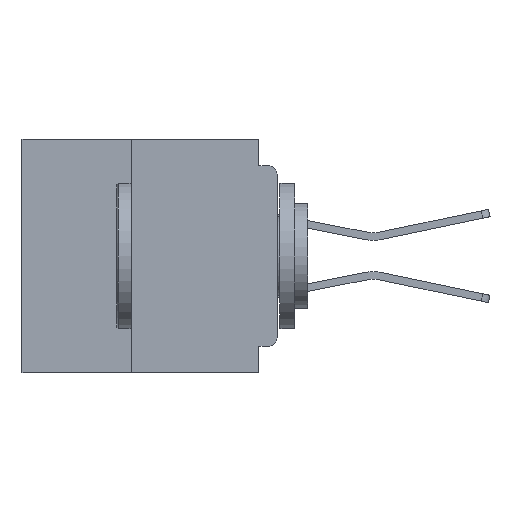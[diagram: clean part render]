
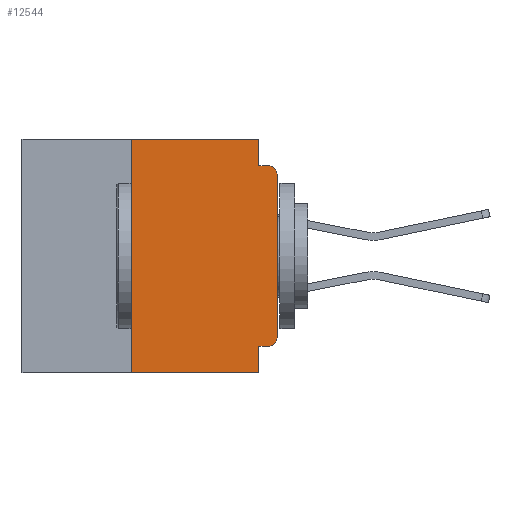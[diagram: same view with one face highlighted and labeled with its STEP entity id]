
A CAD part, left-side view. The second image highlights one B-rep face of the part: STEP entity #12544.
In plain terms, the highlighted planar face has unit normal (-1, 0, 0).
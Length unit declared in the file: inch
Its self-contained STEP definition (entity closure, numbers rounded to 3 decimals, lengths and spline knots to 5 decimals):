
#443 = CARTESIAN_POINT ( 'NONE',  ( 0., 0.015, -0.045 ) ) ;
#712 = LINE ( 'NONE', #4609, #33017 ) ;
#1486 = VECTOR ( 'NONE', #48933, 39.37008 ) ;
#1569 = VERTEX_POINT ( 'NONE', #37169 ) ;
#1986 = LINE ( 'NONE', #53077, #34319 ) ;
#2642 = ORIENTED_EDGE ( 'NONE', *, *, #38864, .F. ) ;
#3159 = CARTESIAN_POINT ( 'NONE',  ( 0., 0.25, -0.4 ) ) ;
#4357 = EDGE_CURVE ( 'NONE', #14208, #6623, #23894, .T. ) ;
#4609 = CARTESIAN_POINT ( 'NONE',  ( 0., 0., -0.045 ) ) ;
#4892 = VECTOR ( 'NONE', #44281, 39.37008 ) ;
#4979 = PLANE ( 'NONE',  #53976 ) ;
#5195 = CARTESIAN_POINT ( 'NONE',  ( 0., 0.031, -0.4 ) ) ;
#5841 = LINE ( 'NONE', #3159, #26900 ) ;
#6285 = LINE ( 'NONE', #45134, #27344 ) ;
#6504 = DIRECTION ( 'NONE',  ( 0., -1., 0. ) ) ;
#6623 = VERTEX_POINT ( 'NONE', #23574 ) ;
#7063 = CARTESIAN_POINT ( 'NONE',  ( 0., 0.031, -0.045 ) ) ;
#9171 = DIRECTION ( 'NONE',  ( -1., 0., 0. ) ) ;
#9175 = DIRECTION ( 'NONE',  ( 1., 0., 0. ) ) ;
#9503 = AXIS2_PLACEMENT_3D ( 'NONE', #43676, #18572, #47808 ) ;
#9841 = VERTEX_POINT ( 'NONE', #47493 ) ;
#10093 = CIRCLE ( 'NONE', #31548, 0.015 ) ;
#10933 = LINE ( 'NONE', #52567, #20792 ) ;
#11069 = ORIENTED_EDGE ( 'NONE', *, *, #26938, .F. ) ;
#12544 = ADVANCED_FACE ( 'NONE', ( #17774 ), #4979, .F. ) ;
#14208 = VERTEX_POINT ( 'NONE', #30816 ) ;
#14665 = ORIENTED_EDGE ( 'NONE', *, *, #43760, .T. ) ;
#15683 = DIRECTION ( 'NONE',  ( 0., 0., -1. ) ) ;
#16078 = LINE ( 'NONE', #40125, #4892 ) ;
#16289 = EDGE_CURVE ( 'NONE', #6623, #36431, #1986, .T. ) ;
#17478 = CARTESIAN_POINT ( 'NONE',  ( 0., 0.437, 0. ) ) ;
#17774 = FACE_OUTER_BOUND ( 'NONE', #49546, .T. ) ;
#18572 = DIRECTION ( 'NONE',  ( -1., 0., 0. ) ) ;
#19112 = EDGE_CURVE ( 'NONE', #25032, #36431, #6285, .T. ) ;
#19873 = VERTEX_POINT ( 'NONE', #40147 ) ;
#20771 = VECTOR ( 'NONE', #49177, 39.37008 ) ;
#20792 = VECTOR ( 'NONE', #6504, 39.37008 ) ;
#21109 = ORIENTED_EDGE ( 'NONE', *, *, #19112, .T. ) ;
#21934 = EDGE_CURVE ( 'NONE', #25032, #9841, #5841, .T. ) ;
#23282 = ORIENTED_EDGE ( 'NONE', *, *, #16289, .F. ) ;
#23304 = VERTEX_POINT ( 'NONE', #7063 ) ;
#23505 = VERTEX_POINT ( 'NONE', #33601 ) ;
#23574 = CARTESIAN_POINT ( 'NONE',  ( 0., 0.031, -0.355 ) ) ;
#23894 = LINE ( 'NONE', #48626, #1486 ) ;
#25032 = VERTEX_POINT ( 'NONE', #39256 ) ;
#26232 = ORIENTED_EDGE ( 'NONE', *, *, #39261, .T. ) ;
#26900 = VECTOR ( 'NONE', #36875, 39.37008 ) ;
#26938 = EDGE_CURVE ( 'NONE', #23304, #48248, #712, .T. ) ;
#27344 = VECTOR ( 'NONE', #53385, 39.37008 ) ;
#28091 = ORIENTED_EDGE ( 'NONE', *, *, #4357, .F. ) ;
#28679 = CIRCLE ( 'NONE', #9503, 0.015 ) ;
#29111 = ORIENTED_EDGE ( 'NONE', *, *, #44802, .T. ) ;
#29619 = ORIENTED_EDGE ( 'NONE', *, *, #21934, .F. ) ;
#30816 = CARTESIAN_POINT ( 'NONE',  ( 0., 0.015, -0.355 ) ) ;
#31548 = AXIS2_PLACEMENT_3D ( 'NONE', #34469, #9171, #38644 ) ;
#33017 = VECTOR ( 'NONE', #34122, 39.37008 ) ;
#33601 = CARTESIAN_POINT ( 'NONE',  ( 0., 0., -0.34 ) ) ;
#34122 = DIRECTION ( 'NONE',  ( 0., -1., 0. ) ) ;
#34319 = VECTOR ( 'NONE', #15683, 39.37008 ) ;
#34469 = CARTESIAN_POINT ( 'NONE',  ( 0., 0.015, -0.34 ) ) ;
#36431 = VERTEX_POINT ( 'NONE', #5195 ) ;
#36875 = DIRECTION ( 'NONE',  ( 0., 0., 1. ) ) ;
#37169 = CARTESIAN_POINT ( 'NONE',  ( 0., 0., -0.06 ) ) ;
#38644 = DIRECTION ( 'NONE',  ( 0., 0., -1. ) ) ;
#38653 = DIRECTION ( 'NONE',  ( 0., 0., -1. ) ) ;
#38864 = EDGE_CURVE ( 'NONE', #19873, #23304, #16078, .T. ) ;
#39256 = CARTESIAN_POINT ( 'NONE',  ( 0., 0.25, -0.4 ) ) ;
#39261 = EDGE_CURVE ( 'NONE', #14208, #23505, #10093, .T. ) ;
#40125 = CARTESIAN_POINT ( 'NONE',  ( 0., 0.031, 0. ) ) ;
#40147 = CARTESIAN_POINT ( 'NONE',  ( 0., 0.031, 0. ) ) ;
#43100 = LINE ( 'NONE', #53498, #20771 ) ;
#43676 = CARTESIAN_POINT ( 'NONE',  ( 0., 0.015, -0.06 ) ) ;
#43760 = EDGE_CURVE ( 'NONE', #23505, #1569, #43100, .T. ) ;
#44281 = DIRECTION ( 'NONE',  ( 0., 0., -1. ) ) ;
#44802 = EDGE_CURVE ( 'NONE', #1569, #48248, #28679, .T. ) ;
#45134 = CARTESIAN_POINT ( 'NONE',  ( 0., 0.437, -0.4 ) ) ;
#46606 = EDGE_CURVE ( 'NONE', #9841, #19873, #10933, .T. ) ;
#47493 = CARTESIAN_POINT ( 'NONE',  ( 0., 0.25, 0. ) ) ;
#47808 = DIRECTION ( 'NONE',  ( 0., 0., -1. ) ) ;
#48248 = VERTEX_POINT ( 'NONE', #443 ) ;
#48626 = CARTESIAN_POINT ( 'NONE',  ( 0., 0., -0.355 ) ) ;
#48933 = DIRECTION ( 'NONE',  ( 0., 1., 0. ) ) ;
#49177 = DIRECTION ( 'NONE',  ( 0., 0., 1. ) ) ;
#49546 = EDGE_LOOP ( 'NONE', ( #14665, #29111, #11069, #2642, #52113, #29619, #21109, #23282, #28091, #26232 ) ) ;
#52113 = ORIENTED_EDGE ( 'NONE', *, *, #46606, .F. ) ;
#52567 = CARTESIAN_POINT ( 'NONE',  ( 0., 0.437, 0. ) ) ;
#53077 = CARTESIAN_POINT ( 'NONE',  ( 0., 0.031, -0.4 ) ) ;
#53385 = DIRECTION ( 'NONE',  ( 0., -1., 0. ) ) ;
#53498 = CARTESIAN_POINT ( 'NONE',  ( 0., 0., 0. ) ) ;
#53976 = AXIS2_PLACEMENT_3D ( 'NONE', #17478, #9175, #38653 ) ;
